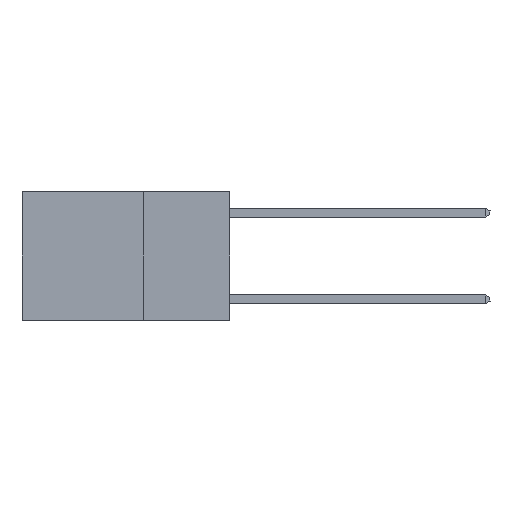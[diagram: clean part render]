
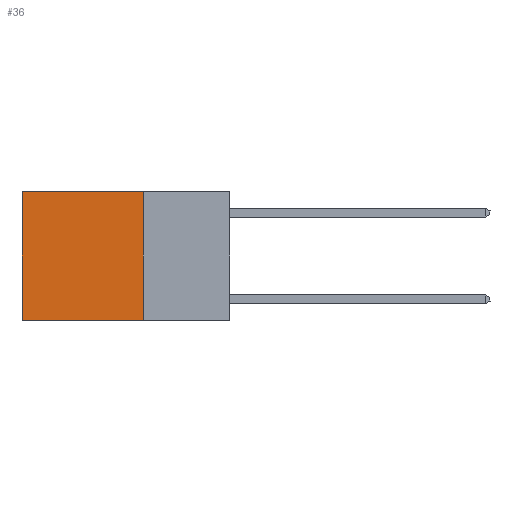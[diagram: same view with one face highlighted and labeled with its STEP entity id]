
A CAD part, left-side view. The second image highlights one B-rep face of the part: STEP entity #36.
In plain terms, the highlighted planar face has unit normal (-1, 0, 0).
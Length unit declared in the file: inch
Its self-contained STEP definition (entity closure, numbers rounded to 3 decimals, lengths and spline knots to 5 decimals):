
#36 = ADVANCED_FACE ( 'NONE', ( #13565 ), #18784, .F. ) ;
#839 = LINE ( 'NONE', #2418, #4005 ) ;
#1902 = ORIENTED_EDGE ( 'NONE', *, *, #18175, .F. ) ;
#1911 = DIRECTION ( 'NONE',  ( 0., 0., -1. ) ) ;
#2418 = CARTESIAN_POINT ( 'NONE',  ( 0.2625, 0.25, -0.37 ) ) ;
#2602 = VERTEX_POINT ( 'NONE', #14058 ) ;
#3210 = LINE ( 'NONE', #15365, #5692 ) ;
#3359 = AXIS2_PLACEMENT_3D ( 'NONE', #15661, #19723, #1911 ) ;
#4005 = VECTOR ( 'NONE', #7148, 39.37008 ) ;
#4436 = CARTESIAN_POINT ( 'NONE',  ( 0.2625, 0.25, 0. ) ) ;
#4939 = VERTEX_POINT ( 'NONE', #11703 ) ;
#5239 = ORIENTED_EDGE ( 'NONE', *, *, #11119, .T. ) ;
#5692 = VECTOR ( 'NONE', #12361, 39.37008 ) ;
#5729 = CARTESIAN_POINT ( 'NONE',  ( 0.2625, 0.25, -0.37 ) ) ;
#6514 = VECTOR ( 'NONE', #19332, 39.37008 ) ;
#6758 = VERTEX_POINT ( 'NONE', #5729 ) ;
#7148 = DIRECTION ( 'NONE',  ( 0., 1., 0. ) ) ;
#8500 = ORIENTED_EDGE ( 'NONE', *, *, #18963, .T. ) ;
#10256 = DIRECTION ( 'NONE',  ( 0., 0., -1. ) ) ;
#11119 = EDGE_CURVE ( 'NONE', #2602, #4939, #15054, .T. ) ;
#11703 = CARTESIAN_POINT ( 'NONE',  ( 0.2625, 0.6, -0.37 ) ) ;
#12361 = DIRECTION ( 'NONE',  ( 0., 0., -1. ) ) ;
#12577 = ORIENTED_EDGE ( 'NONE', *, *, #18523, .F. ) ;
#12895 = CARTESIAN_POINT ( 'NONE',  ( 0.2625, 0.25, 0. ) ) ;
#13565 = FACE_OUTER_BOUND ( 'NONE', #15327, .T. ) ;
#14058 = CARTESIAN_POINT ( 'NONE',  ( 0.2625, 0.6, 0. ) ) ;
#15054 = LINE ( 'NONE', #15268, #19809 ) ;
#15268 = CARTESIAN_POINT ( 'NONE',  ( 0.2625, 0.6, 0. ) ) ;
#15327 = EDGE_LOOP ( 'NONE', ( #5239, #1902, #12577, #8500 ) ) ;
#15365 = CARTESIAN_POINT ( 'NONE',  ( 0.2625, 0.25, 0. ) ) ;
#15661 = CARTESIAN_POINT ( 'NONE',  ( 0.2625, 0.25, 0. ) ) ;
#17964 = VERTEX_POINT ( 'NONE', #4436 ) ;
#18175 = EDGE_CURVE ( 'NONE', #6758, #4939, #839, .T. ) ;
#18523 = EDGE_CURVE ( 'NONE', #17964, #6758, #3210, .T. ) ;
#18784 = PLANE ( 'NONE',  #3359 ) ;
#18963 = EDGE_CURVE ( 'NONE', #17964, #2602, #19234, .T. ) ;
#19234 = LINE ( 'NONE', #12895, #6514 ) ;
#19332 = DIRECTION ( 'NONE',  ( 0., 1., 0. ) ) ;
#19723 = DIRECTION ( 'NONE',  ( 1., 0., 0. ) ) ;
#19809 = VECTOR ( 'NONE', #10256, 39.37008 ) ;
